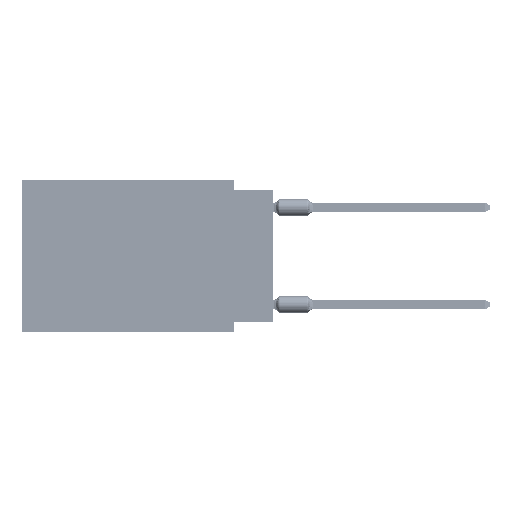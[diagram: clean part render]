
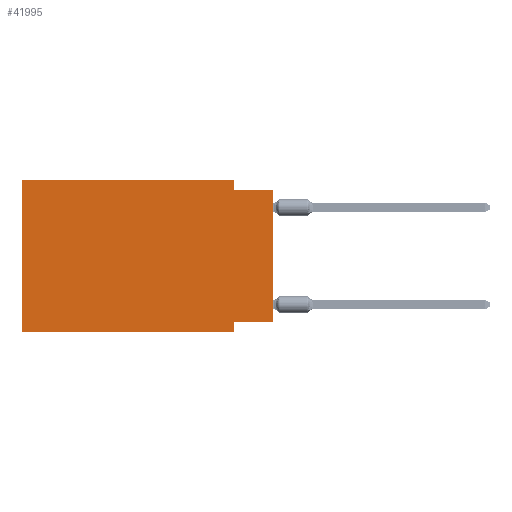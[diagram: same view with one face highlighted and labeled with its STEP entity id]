
A CAD part, left-side view. The second image highlights one B-rep face of the part: STEP entity #41995.
In plain terms, the highlighted planar face has unit normal (-1, 0, 0).
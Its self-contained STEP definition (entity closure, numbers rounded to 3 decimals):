
#91 = ORIENTED_EDGE ( 'NONE', *, *, #19229, .F. ) ;
#966 = EDGE_CURVE ( 'NONE', #24804, #63904, #32197, .T. ) ;
#1224 = CARTESIAN_POINT ( 'NONE',  ( 0., 2.54, -0.635 ) ) ;
#2085 = CARTESIAN_POINT ( 'NONE',  ( 0., 0., -9.271 ) ) ;
#4332 = ORIENTED_EDGE ( 'NONE', *, *, #13429, .F. ) ;
#4943 = AXIS2_PLACEMENT_3D ( 'NONE', #75241, #51737, #51353 ) ;
#5493 = VERTEX_POINT ( 'NONE', #40265 ) ;
#5945 = LINE ( 'NONE', #72893, #22286 ) ;
#9487 = LINE ( 'NONE', #2085, #47478 ) ;
#12560 = VECTOR ( 'NONE', #70326, 1000. ) ;
#13429 = EDGE_CURVE ( 'NONE', #30256, #65665, #24406, .T. ) ;
#14380 = DIRECTION ( 'NONE',  ( 0., 0., 1. ) ) ;
#15408 = EDGE_CURVE ( 'NONE', #65665, #24804, #5945, .T. ) ;
#15498 = VECTOR ( 'NONE', #59999, 1000. ) ;
#18757 = CARTESIAN_POINT ( 'NONE',  ( 0., 16.383, 0. ) ) ;
#19229 = EDGE_CURVE ( 'NONE', #25390, #5493, #9487, .T. ) ;
#20919 = ORIENTED_EDGE ( 'NONE', *, *, #966, .F. ) ;
#22286 = VECTOR ( 'NONE', #54097, 1000. ) ;
#22608 = LINE ( 'NONE', #46466, #12560 ) ;
#24406 = LINE ( 'NONE', #72549, #64353 ) ;
#24642 = LINE ( 'NONE', #29735, #55888 ) ;
#24804 = VERTEX_POINT ( 'NONE', #72222 ) ;
#25390 = VERTEX_POINT ( 'NONE', #69214 ) ;
#26166 = LINE ( 'NONE', #44528, #65070 ) ;
#29735 = CARTESIAN_POINT ( 'NONE',  ( 0., 2.54, -9.906 ) ) ;
#29894 = LINE ( 'NONE', #36165, #15498 ) ;
#30256 = VERTEX_POINT ( 'NONE', #41070 ) ;
#30661 = ORIENTED_EDGE ( 'NONE', *, *, #35810, .F. ) ;
#32197 = LINE ( 'NONE', #68926, #45269 ) ;
#33764 = FACE_OUTER_BOUND ( 'NONE', #39440, .T. ) ;
#35810 = EDGE_CURVE ( 'NONE', #63904, #37195, #22608, .T. ) ;
#36165 = CARTESIAN_POINT ( 'NONE',  ( 0., 16.383, -9.906 ) ) ;
#37195 = VERTEX_POINT ( 'NONE', #58821 ) ;
#37328 = DIRECTION ( 'NONE',  ( 0., 0., 1. ) ) ;
#38551 = EDGE_CURVE ( 'NONE', #30256, #48155, #29894, .T. ) ;
#39440 = EDGE_LOOP ( 'NONE', ( #72424, #30661, #20919, #44676, #4332, #57080, #47703, #91 ) ) ;
#40265 = CARTESIAN_POINT ( 'NONE',  ( 0., 2.54, -9.271 ) ) ;
#41070 = CARTESIAN_POINT ( 'NONE',  ( 0., 16.383, -9.906 ) ) ;
#41995 = ADVANCED_FACE ( 'NONE', ( #33764 ), #70504, .F. ) ;
#42696 = EDGE_CURVE ( 'NONE', #25390, #37195, #26166, .T. ) ;
#44528 = CARTESIAN_POINT ( 'NONE',  ( 0., 0., 0. ) ) ;
#44676 = ORIENTED_EDGE ( 'NONE', *, *, #15408, .F. ) ;
#45269 = VECTOR ( 'NONE', #68548, 1000. ) ;
#46466 = CARTESIAN_POINT ( 'NONE',  ( 0., 0., -0.635 ) ) ;
#47478 = VECTOR ( 'NONE', #56860, 1000. ) ;
#47703 = ORIENTED_EDGE ( 'NONE', *, *, #62509, .F. ) ;
#48155 = VERTEX_POINT ( 'NONE', #59074 ) ;
#51353 = DIRECTION ( 'NONE',  ( 0., 0., -1. ) ) ;
#51737 = DIRECTION ( 'NONE',  ( 1., 0., 0. ) ) ;
#54097 = DIRECTION ( 'NONE',  ( 0., -1., 0. ) ) ;
#55888 = VECTOR ( 'NONE', #77099, 1000. ) ;
#56860 = DIRECTION ( 'NONE',  ( 0., 1., 0. ) ) ;
#57080 = ORIENTED_EDGE ( 'NONE', *, *, #38551, .T. ) ;
#58821 = CARTESIAN_POINT ( 'NONE',  ( 0., 0., -0.635 ) ) ;
#59074 = CARTESIAN_POINT ( 'NONE',  ( 0., 2.54, -9.906 ) ) ;
#59999 = DIRECTION ( 'NONE',  ( 0., -1., 0. ) ) ;
#62509 = EDGE_CURVE ( 'NONE', #5493, #48155, #24642, .T. ) ;
#63904 = VERTEX_POINT ( 'NONE', #1224 ) ;
#64353 = VECTOR ( 'NONE', #37328, 1000. ) ;
#65070 = VECTOR ( 'NONE', #14380, 1000. ) ;
#65665 = VERTEX_POINT ( 'NONE', #18757 ) ;
#68548 = DIRECTION ( 'NONE',  ( 0., 0., -1. ) ) ;
#68926 = CARTESIAN_POINT ( 'NONE',  ( 0., 2.54, 0. ) ) ;
#69214 = CARTESIAN_POINT ( 'NONE',  ( 0., 0., -9.271 ) ) ;
#70326 = DIRECTION ( 'NONE',  ( 0., -1., 0. ) ) ;
#70504 = PLANE ( 'NONE',  #4943 ) ;
#72222 = CARTESIAN_POINT ( 'NONE',  ( 0., 2.54, 0. ) ) ;
#72424 = ORIENTED_EDGE ( 'NONE', *, *, #42696, .T. ) ;
#72549 = CARTESIAN_POINT ( 'NONE',  ( 0., 16.383, 0. ) ) ;
#72893 = CARTESIAN_POINT ( 'NONE',  ( 0., 16.383, 0. ) ) ;
#75241 = CARTESIAN_POINT ( 'NONE',  ( 0., 16.383, 0. ) ) ;
#77099 = DIRECTION ( 'NONE',  ( 0., 0., -1. ) ) ;
